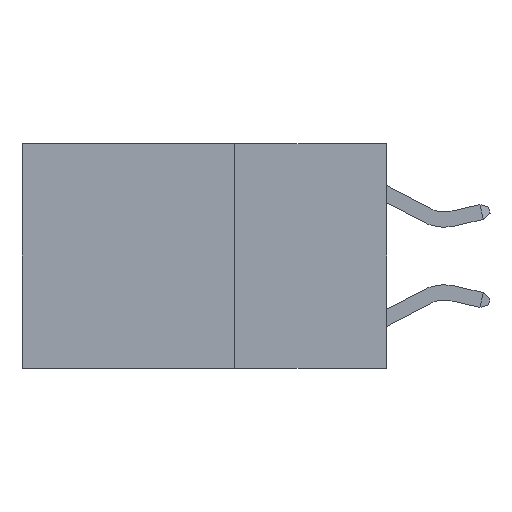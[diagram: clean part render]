
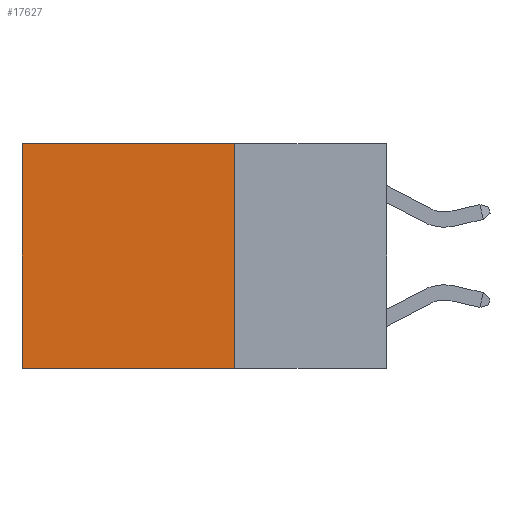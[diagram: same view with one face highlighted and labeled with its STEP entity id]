
A CAD part, left-side view. The second image highlights one B-rep face of the part: STEP entity #17627.
In plain terms, the highlighted planar face has unit normal (-1, 0, 0).
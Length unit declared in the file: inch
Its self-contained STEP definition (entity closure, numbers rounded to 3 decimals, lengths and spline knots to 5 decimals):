
#1142 = DIRECTION ( 'NONE',  ( 0., 0., -1. ) ) ;
#2011 = LINE ( 'NONE', #21044, #12426 ) ;
#2042 = VERTEX_POINT ( 'NONE', #2935 ) ;
#2474 = VECTOR ( 'NONE', #15267, 39.37008 ) ;
#2818 = VERTEX_POINT ( 'NONE', #6971 ) ;
#2935 = CARTESIAN_POINT ( 'NONE',  ( 0.2625, 0.6, -0.37 ) ) ;
#3057 = CARTESIAN_POINT ( 'NONE',  ( 0.2625, 0.6, 0. ) ) ;
#3106 = LINE ( 'NONE', #13302, #2474 ) ;
#3578 = ORIENTED_EDGE ( 'NONE', *, *, #19408, .T. ) ;
#4997 = CARTESIAN_POINT ( 'NONE',  ( 0.2625, 0.25, -0.37 ) ) ;
#5519 = DIRECTION ( 'NONE',  ( 0., 0., -1. ) ) ;
#6432 = VECTOR ( 'NONE', #13831, 39.37008 ) ;
#6971 = CARTESIAN_POINT ( 'NONE',  ( 0.2625, 0.25, 0. ) ) ;
#7054 = LINE ( 'NONE', #15726, #6432 ) ;
#7757 = ORIENTED_EDGE ( 'NONE', *, *, #20824, .F. ) ;
#9491 = DIRECTION ( 'NONE',  ( 0., 1., 0. ) ) ;
#9583 = ORIENTED_EDGE ( 'NONE', *, *, #24410, .T. ) ;
#10226 = VERTEX_POINT ( 'NONE', #4997 ) ;
#11311 = PLANE ( 'NONE',  #11430 ) ;
#11430 = AXIS2_PLACEMENT_3D ( 'NONE', #24682, #17171, #5519 ) ;
#12288 = CARTESIAN_POINT ( 'NONE',  ( 0.2625, 0.6, 0. ) ) ;
#12426 = VECTOR ( 'NONE', #9491, 39.37008 ) ;
#12702 = VERTEX_POINT ( 'NONE', #12288 ) ;
#12896 = ORIENTED_EDGE ( 'NONE', *, *, #24563, .F. ) ;
#13302 = CARTESIAN_POINT ( 'NONE',  ( 0.2625, 0.25, 0. ) ) ;
#13831 = DIRECTION ( 'NONE',  ( 0., 0., -1. ) ) ;
#15267 = DIRECTION ( 'NONE',  ( 0., 1., 0. ) ) ;
#15497 = VECTOR ( 'NONE', #1142, 39.37008 ) ;
#15726 = CARTESIAN_POINT ( 'NONE',  ( 0.2625, 0.25, 0. ) ) ;
#16317 = FACE_OUTER_BOUND ( 'NONE', #18332, .T. ) ;
#17171 = DIRECTION ( 'NONE',  ( 1., 0., 0. ) ) ;
#17627 = ADVANCED_FACE ( 'NONE', ( #16317 ), #11311, .F. ) ;
#18332 = EDGE_LOOP ( 'NONE', ( #9583, #12896, #7757, #3578 ) ) ;
#19408 = EDGE_CURVE ( 'NONE', #2818, #12702, #3106, .T. ) ;
#20596 = LINE ( 'NONE', #3057, #15497 ) ;
#20824 = EDGE_CURVE ( 'NONE', #2818, #10226, #7054, .T. ) ;
#21044 = CARTESIAN_POINT ( 'NONE',  ( 0.2625, 0.25, -0.37 ) ) ;
#24410 = EDGE_CURVE ( 'NONE', #12702, #2042, #20596, .T. ) ;
#24563 = EDGE_CURVE ( 'NONE', #10226, #2042, #2011, .T. ) ;
#24682 = CARTESIAN_POINT ( 'NONE',  ( 0.2625, 0.25, 0. ) ) ;
